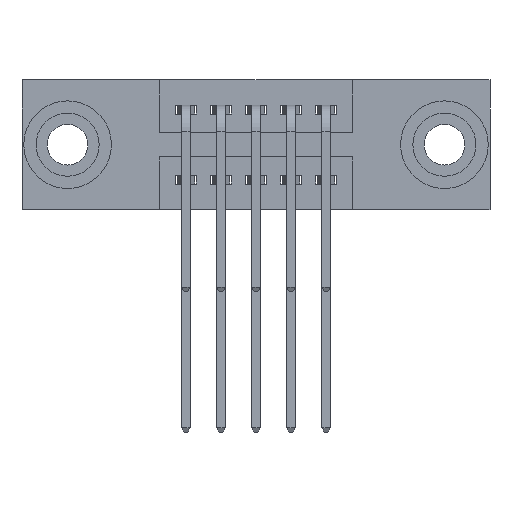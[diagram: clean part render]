
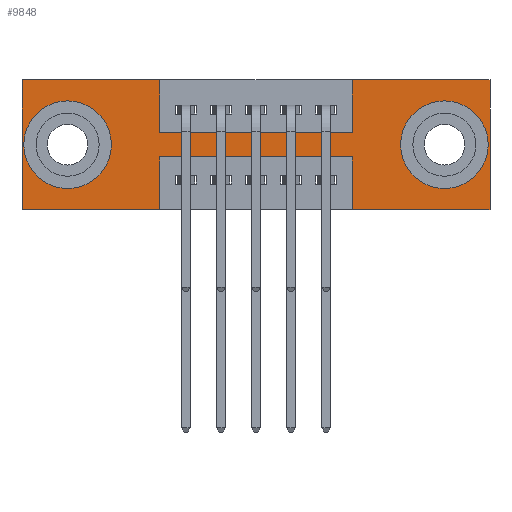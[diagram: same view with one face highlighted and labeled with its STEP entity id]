
A CAD part, front view. The second image highlights one B-rep face of the part: STEP entity #9848.
In plain terms, the highlighted planar face has unit normal (0, -1, 0).
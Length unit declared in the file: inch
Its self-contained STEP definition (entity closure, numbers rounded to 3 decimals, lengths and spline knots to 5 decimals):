
#21 = VERTEX_POINT ( 'NONE', #9420 ) ;
#132 = VECTOR ( 'NONE', #9560, 39.37008 ) ;
#229 = VECTOR ( 'NONE', #5400, 39.37008 ) ;
#447 = DIRECTION ( 'NONE',  ( 0., -1., 0. ) ) ;
#659 = ORIENTED_EDGE ( 'NONE', *, *, #4693, .F. ) ;
#693 = EDGE_CURVE ( 'NONE', #5625, #5839, #9468, .T. ) ;
#913 = CARTESIAN_POINT ( 'NONE',  ( 0., 0., 0. ) ) ;
#1202 = VERTEX_POINT ( 'NONE', #6675 ) ;
#1227 = ORIENTED_EDGE ( 'NONE', *, *, #1919, .F. ) ;
#1364 = AXIS2_PLACEMENT_3D ( 'NONE', #8415, #6798, #3390 ) ;
#1528 = ORIENTED_EDGE ( 'NONE', *, *, #1761, .F. ) ;
#1536 = ORIENTED_EDGE ( 'NONE', *, *, #10688, .T. ) ;
#1742 = VERTEX_POINT ( 'NONE', #8428 ) ;
#1761 = EDGE_CURVE ( 'NONE', #5839, #5731, #10141, .T. ) ;
#1844 = CARTESIAN_POINT ( 'NONE',  ( 0.9425, 0., -0.37 ) ) ;
#1866 = EDGE_CURVE ( 'NONE', #6013, #5152, #5153, .T. ) ;
#1919 = EDGE_CURVE ( 'NONE', #5152, #8054, #3399, .T. ) ;
#1934 = ORIENTED_EDGE ( 'NONE', *, *, #6083, .F. ) ;
#1980 = VECTOR ( 'NONE', #5583, 39.37008 ) ;
#2146 = VERTEX_POINT ( 'NONE', #7513 ) ;
#2217 = LINE ( 'NONE', #5314, #2631 ) ;
#2248 = ORIENTED_EDGE ( 'NONE', *, *, #9195, .T. ) ;
#2265 = PLANE ( 'NONE',  #3977 ) ;
#2278 = DIRECTION ( 'NONE',  ( 0., 0., -1. ) ) ;
#2356 = LINE ( 'NONE', #4625, #8833 ) ;
#2415 = ORIENTED_EDGE ( 'NONE', *, *, #5952, .F. ) ;
#2474 = CARTESIAN_POINT ( 'NONE',  ( 0.13, 0., -0.263 ) ) ;
#2509 = EDGE_CURVE ( 'NONE', #1202, #5625, #9837, .T. ) ;
#2631 = VECTOR ( 'NONE', #2718, 39.37008 ) ;
#2718 = DIRECTION ( 'NONE',  ( 0., 0., -1. ) ) ;
#2789 = CARTESIAN_POINT ( 'NONE',  ( 0., 0., -0.37 ) ) ;
#2903 = FACE_BOUND ( 'NONE', #8821, .T. ) ;
#2979 = CARTESIAN_POINT ( 'NONE',  ( 1.335, 0., -0.37 ) ) ;
#2999 = VERTEX_POINT ( 'NONE', #10615 ) ;
#3005 = DIRECTION ( 'NONE',  ( 0., 1., 0. ) ) ;
#3254 = DIRECTION ( 'NONE',  ( 0., 1., 0. ) ) ;
#3390 = DIRECTION ( 'NONE',  ( 0., 0., 1. ) ) ;
#3399 = LINE ( 'NONE', #1844, #10400 ) ;
#3569 = EDGE_CURVE ( 'NONE', #10706, #6887, #6978, .T. ) ;
#3597 = CARTESIAN_POINT ( 'NONE',  ( 0., 0., 0. ) ) ;
#3672 = EDGE_CURVE ( 'NONE', #2146, #2999, #10636, .T. ) ;
#3713 = CIRCLE ( 'NONE', #8407, 0.078 ) ;
#3755 = ORIENTED_EDGE ( 'NONE', *, *, #3672, .T. ) ;
#3781 = CARTESIAN_POINT ( 'NONE',  ( 0.9425, 0., 0. ) ) ;
#3787 = DIRECTION ( 'NONE',  ( 1., 0., 0. ) ) ;
#3947 = LINE ( 'NONE', #6301, #9435 ) ;
#3977 = AXIS2_PLACEMENT_3D ( 'NONE', #10857, #447, #8159 ) ;
#4435 = CARTESIAN_POINT ( 'NONE',  ( 1.205, 0., -0.185 ) ) ;
#4549 = VERTEX_POINT ( 'NONE', #9553 ) ;
#4625 = CARTESIAN_POINT ( 'NONE',  ( 0.3925, 0., -0.37 ) ) ;
#4693 = EDGE_CURVE ( 'NONE', #1742, #1202, #2356, .T. ) ;
#4825 = AXIS2_PLACEMENT_3D ( 'NONE', #6711, #3254, #2278 ) ;
#5008 = ORIENTED_EDGE ( 'NONE', *, *, #5934, .F. ) ;
#5026 = VECTOR ( 'NONE', #7033, 39.37008 ) ;
#5101 = ORIENTED_EDGE ( 'NONE', *, *, #3569, .F. ) ;
#5150 = LINE ( 'NONE', #5969, #11189 ) ;
#5152 = VERTEX_POINT ( 'NONE', #5183 ) ;
#5153 = LINE ( 'NONE', #2789, #7949 ) ;
#5183 = CARTESIAN_POINT ( 'NONE',  ( 0.9425, 0., -0.37 ) ) ;
#5196 = FACE_BOUND ( 'NONE', #10143, .T. ) ;
#5254 = ORIENTED_EDGE ( 'NONE', *, *, #8835, .F. ) ;
#5308 = DIRECTION ( 'NONE',  ( 0., 0., -1. ) ) ;
#5314 = CARTESIAN_POINT ( 'NONE',  ( 0.3925, 0., 0. ) ) ;
#5359 = ORIENTED_EDGE ( 'NONE', *, *, #1866, .F. ) ;
#5400 = DIRECTION ( 'NONE',  ( -1., 0., 0. ) ) ;
#5416 = DIRECTION ( 'NONE',  ( 0., 0., -1. ) ) ;
#5552 = LINE ( 'NONE', #8774, #8600 ) ;
#5583 = DIRECTION ( 'NONE',  ( 0., 0., 1. ) ) ;
#5625 = VERTEX_POINT ( 'NONE', #5918 ) ;
#5731 = VERTEX_POINT ( 'NONE', #7028 ) ;
#5839 = VERTEX_POINT ( 'NONE', #8118 ) ;
#5866 = FACE_OUTER_BOUND ( 'NONE', #6510, .T. ) ;
#5888 = CARTESIAN_POINT ( 'NONE',  ( 0., 0., -0.37 ) ) ;
#5918 = CARTESIAN_POINT ( 'NONE',  ( 0., 0., -0.37 ) ) ;
#5934 = EDGE_CURVE ( 'NONE', #21, #10706, #3947, .T. ) ;
#5952 = EDGE_CURVE ( 'NONE', #8054, #1742, #9549, .T. ) ;
#5969 = CARTESIAN_POINT ( 'NONE',  ( 0., 0., 0. ) ) ;
#6013 = VERTEX_POINT ( 'NONE', #2979 ) ;
#6083 = EDGE_CURVE ( 'NONE', #6887, #9213, #5150, .T. ) ;
#6203 = DIRECTION ( 'NONE',  ( 0., 0., -1. ) ) ;
#6205 = DIRECTION ( 'NONE',  ( 0., 1., 0. ) ) ;
#6301 = CARTESIAN_POINT ( 'NONE',  ( 0.3925, 0., -0.15 ) ) ;
#6321 = CARTESIAN_POINT ( 'NONE',  ( 1.335, 0., 0. ) ) ;
#6465 = CARTESIAN_POINT ( 'NONE',  ( 0.13, 0., -0.185 ) ) ;
#6510 = EDGE_LOOP ( 'NONE', ( #659, #2415, #1227, #5359, #11231, #1934, #5101, #5008, #5254, #1528, #9287, #10341 ) ) ;
#6675 = CARTESIAN_POINT ( 'NONE',  ( 0.3925, 0., -0.37 ) ) ;
#6688 = CARTESIAN_POINT ( 'NONE',  ( 0.9425, 0., -0.22 ) ) ;
#6711 = CARTESIAN_POINT ( 'NONE',  ( 1.205, 0., -0.185 ) ) ;
#6726 = EDGE_CURVE ( 'NONE', #9213, #6013, #5552, .T. ) ;
#6798 = DIRECTION ( 'NONE',  ( 0., 1., 0. ) ) ;
#6887 = VERTEX_POINT ( 'NONE', #8124 ) ;
#6978 = LINE ( 'NONE', #3781, #1980 ) ;
#7028 = CARTESIAN_POINT ( 'NONE',  ( 0.3925, 0., 0. ) ) ;
#7033 = DIRECTION ( 'NONE',  ( 1., 0., 0. ) ) ;
#7046 = DIRECTION ( 'NONE',  ( 1., 0., 0. ) ) ;
#7083 = EDGE_CURVE ( 'NONE', #4549, #10765, #9972, .T. ) ;
#7513 = CARTESIAN_POINT ( 'NONE',  ( 1.205, 0., -0.263 ) ) ;
#7599 = DIRECTION ( 'NONE',  ( -1., 0., 0. ) ) ;
#7630 = DIRECTION ( 'NONE',  ( -1., 0., 0. ) ) ;
#7949 = VECTOR ( 'NONE', #7630, 39.37008 ) ;
#8054 = VERTEX_POINT ( 'NONE', #6688 ) ;
#8118 = CARTESIAN_POINT ( 'NONE',  ( 0., 0., 0. ) ) ;
#8124 = CARTESIAN_POINT ( 'NONE',  ( 0.9425, 0., 0. ) ) ;
#8159 = DIRECTION ( 'NONE',  ( 0., 0., -1. ) ) ;
#8407 = AXIS2_PLACEMENT_3D ( 'NONE', #4435, #6205, #5308 ) ;
#8415 = CARTESIAN_POINT ( 'NONE',  ( 0.13, 0., -0.185 ) ) ;
#8428 = CARTESIAN_POINT ( 'NONE',  ( 0.3925, 0., -0.22 ) ) ;
#8600 = VECTOR ( 'NONE', #6203, 39.37008 ) ;
#8774 = CARTESIAN_POINT ( 'NONE',  ( 1.335, 0., 0. ) ) ;
#8821 = EDGE_LOOP ( 'NONE', ( #9894, #2248 ) ) ;
#8833 = VECTOR ( 'NONE', #5416, 39.37008 ) ;
#8835 = EDGE_CURVE ( 'NONE', #5731, #21, #2217, .T. ) ;
#8890 = VECTOR ( 'NONE', #7599, 39.37008 ) ;
#8951 = CARTESIAN_POINT ( 'NONE',  ( 0.3925, 0., -0.22 ) ) ;
#9108 = CIRCLE ( 'NONE', #10345, 0.078 ) ;
#9195 = EDGE_CURVE ( 'NONE', #10765, #4549, #9108, .T. ) ;
#9213 = VERTEX_POINT ( 'NONE', #6321 ) ;
#9287 = ORIENTED_EDGE ( 'NONE', *, *, #693, .F. ) ;
#9420 = CARTESIAN_POINT ( 'NONE',  ( 0.3925, 0., -0.15 ) ) ;
#9435 = VECTOR ( 'NONE', #3787, 39.37008 ) ;
#9468 = LINE ( 'NONE', #913, #132 ) ;
#9532 = DIRECTION ( 'NONE',  ( 0., 0., 1. ) ) ;
#9549 = LINE ( 'NONE', #8951, #229 ) ;
#9553 = CARTESIAN_POINT ( 'NONE',  ( 0.13, 0., -0.107 ) ) ;
#9560 = DIRECTION ( 'NONE',  ( 0., 0., 1. ) ) ;
#9637 = CARTESIAN_POINT ( 'NONE',  ( 0.9425, 0., -0.15 ) ) ;
#9722 = DIRECTION ( 'NONE',  ( 0., 0., 1. ) ) ;
#9837 = LINE ( 'NONE', #5888, #8890 ) ;
#9848 = ADVANCED_FACE ( 'NONE', ( #5196, #2903, #5866 ), #2265, .T. ) ;
#9894 = ORIENTED_EDGE ( 'NONE', *, *, #7083, .T. ) ;
#9972 = CIRCLE ( 'NONE', #1364, 0.078 ) ;
#10141 = LINE ( 'NONE', #3597, #5026 ) ;
#10143 = EDGE_LOOP ( 'NONE', ( #1536, #3755 ) ) ;
#10341 = ORIENTED_EDGE ( 'NONE', *, *, #2509, .F. ) ;
#10345 = AXIS2_PLACEMENT_3D ( 'NONE', #6465, #3005, #9722 ) ;
#10400 = VECTOR ( 'NONE', #9532, 39.37008 ) ;
#10615 = CARTESIAN_POINT ( 'NONE',  ( 1.205, 0., -0.107 ) ) ;
#10636 = CIRCLE ( 'NONE', #4825, 0.078 ) ;
#10688 = EDGE_CURVE ( 'NONE', #2999, #2146, #3713, .T. ) ;
#10706 = VERTEX_POINT ( 'NONE', #9637 ) ;
#10765 = VERTEX_POINT ( 'NONE', #2474 ) ;
#10857 = CARTESIAN_POINT ( 'NONE',  ( 0., 0., -0.37 ) ) ;
#11189 = VECTOR ( 'NONE', #7046, 39.37008 ) ;
#11231 = ORIENTED_EDGE ( 'NONE', *, *, #6726, .F. ) ;
